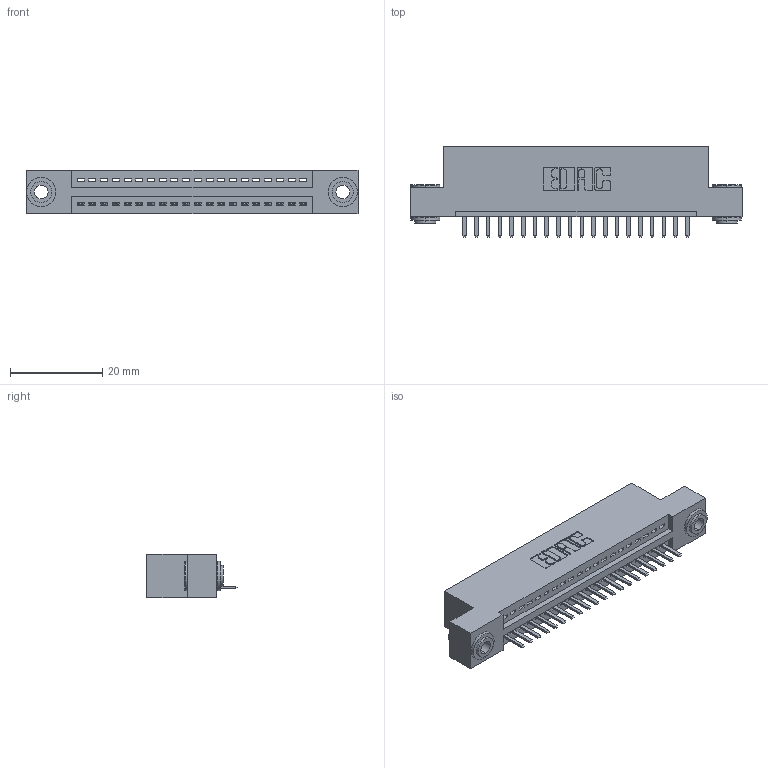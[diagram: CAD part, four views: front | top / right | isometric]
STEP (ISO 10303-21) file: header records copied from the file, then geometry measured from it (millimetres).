
FILE_DESCRIPTION (( 'STEP AP203' ), '1' );
FILE_NAME ('395-020-520-103.STEP', '2019-10-17T18:01:45', ( '' ), ( '' ), 'SwSTEP 2.0', 'SolidWorks 2016', '' );
FILE_SCHEMA (( 'CONFIG_CONTROL_DESIGN' ));
Length unit declared in the file: inch
Products named in the file (4): 345-250-002_345-250-002-102; 395-020-520-103; 345-292-001_345-293-120; 345 Part_Flush Mounting Lugs - 0.156 Dia-TH
Assembly tree (23 placements, depth 2):
  395-020-520-103
    345 Part_Flush Mounting Lugs - 0.156 Dia-TH
    345-292-001_345-293-120  x20
    345-250-002_345-250-002-102  x2
Bounding box: 72.01 x 19.68 x 9.4 mm (x, y, z)
Volume: 6621.1 mm3; surface area: 8526.2 mm2
Topology: 23 solids, 23 shells, 1404 faces, 4097 edges, 2674 vertices
Faces by surface type: plane 930, cylinder 466, cone 8
Entity records: 18778 total; most frequent: CARTESIAN_POINT 3243, ORIENTED_EDGE 3178, DIRECTION 2883, EDGE_CURVE 1589, LINE 1349, VECTOR 1349, VERTEX_POINT 1054, AXIS2_PLACEMENT_3D 767
